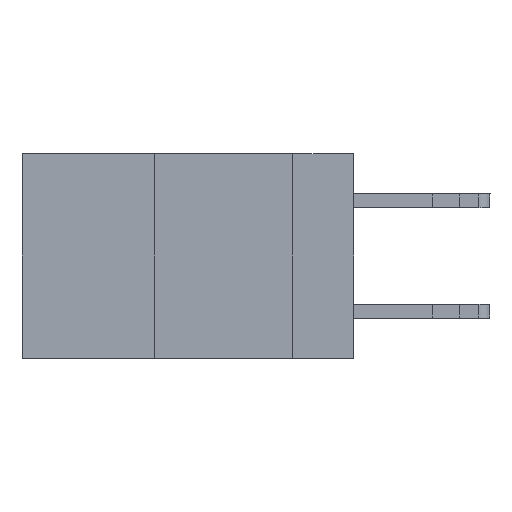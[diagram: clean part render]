
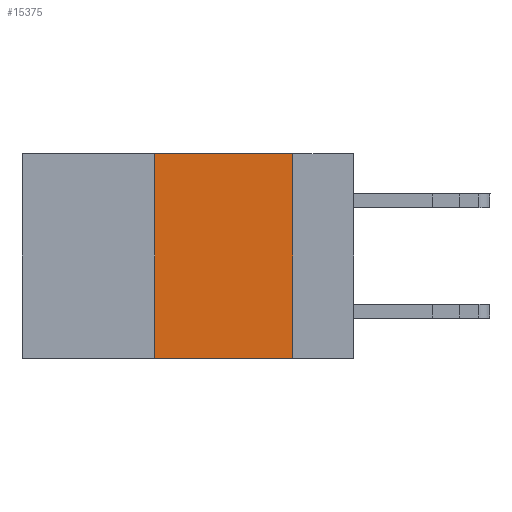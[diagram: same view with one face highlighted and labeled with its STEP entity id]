
A CAD part, left-side view. The second image highlights one B-rep face of the part: STEP entity #15375.
In plain terms, the highlighted planar face has unit normal (-1, 0, 0).
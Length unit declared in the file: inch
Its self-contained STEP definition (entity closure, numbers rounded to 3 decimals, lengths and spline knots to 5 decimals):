
#1478 = EDGE_CURVE ( 'NONE', #24300, #24697, #26715, .T. ) ;
#2427 = EDGE_CURVE ( 'NONE', #22450, #24697, #25152, .T. ) ;
#2754 = CARTESIAN_POINT ( 'NONE',  ( 0., 0.11, 0. ) ) ;
#3565 = PLANE ( 'NONE',  #10828 ) ;
#3780 = DIRECTION ( 'NONE',  ( 1., 0., 0. ) ) ;
#5865 = DIRECTION ( 'NONE',  ( 0., 0., 1. ) ) ;
#6190 = DIRECTION ( 'NONE',  ( 0., 0., -1. ) ) ;
#7989 = VECTOR ( 'NONE', #25671, 39.37008 ) ;
#8071 = ORIENTED_EDGE ( 'NONE', *, *, #12324, .F. ) ;
#8124 = ORIENTED_EDGE ( 'NONE', *, *, #1478, .T. ) ;
#8428 = ORIENTED_EDGE ( 'NONE', *, *, #28635, .F. ) ;
#8718 = VECTOR ( 'NONE', #17264, 39.37008 ) ;
#10828 = AXIS2_PLACEMENT_3D ( 'NONE', #18059, #3780, #6190 ) ;
#11264 = CARTESIAN_POINT ( 'NONE',  ( 0., 0.36, 0. ) ) ;
#11958 = CARTESIAN_POINT ( 'NONE',  ( 0., 0.11, -0.37 ) ) ;
#12175 = CARTESIAN_POINT ( 'NONE',  ( 0., 0.36, 0. ) ) ;
#12324 = EDGE_CURVE ( 'NONE', #24300, #23163, #24740, .T. ) ;
#14173 = EDGE_LOOP ( 'NONE', ( #14242, #8428, #8071, #8124 ) ) ;
#14242 = ORIENTED_EDGE ( 'NONE', *, *, #2427, .F. ) ;
#15375 = ADVANCED_FACE ( 'NONE', ( #24974 ), #3565, .F. ) ;
#16295 = CARTESIAN_POINT ( 'NONE',  ( 0., 0.6, -0.37 ) ) ;
#17264 = DIRECTION ( 'NONE',  ( 0., -1., 0. ) ) ;
#17408 = CARTESIAN_POINT ( 'NONE',  ( 0., 0.36, -0.37 ) ) ;
#18059 = CARTESIAN_POINT ( 'NONE',  ( 0., 0.6, 0. ) ) ;
#18063 = VECTOR ( 'NONE', #22078, 39.37008 ) ;
#18240 = CARTESIAN_POINT ( 'NONE',  ( 0., 0.11, 0. ) ) ;
#22078 = DIRECTION ( 'NONE',  ( 0., 0., -1. ) ) ;
#22450 = VERTEX_POINT ( 'NONE', #18240 ) ;
#23163 = VERTEX_POINT ( 'NONE', #11264 ) ;
#24300 = VERTEX_POINT ( 'NONE', #17408 ) ;
#24556 = CARTESIAN_POINT ( 'NONE',  ( 0., 0.6, 0. ) ) ;
#24697 = VERTEX_POINT ( 'NONE', #11958 ) ;
#24740 = LINE ( 'NONE', #12175, #28860 ) ;
#24974 = FACE_OUTER_BOUND ( 'NONE', #14173, .T. ) ;
#25152 = LINE ( 'NONE', #2754, #18063 ) ;
#25597 = LINE ( 'NONE', #24556, #8718 ) ;
#25671 = DIRECTION ( 'NONE',  ( 0., -1., 0. ) ) ;
#26715 = LINE ( 'NONE', #16295, #7989 ) ;
#28635 = EDGE_CURVE ( 'NONE', #23163, #22450, #25597, .T. ) ;
#28860 = VECTOR ( 'NONE', #5865, 39.37008 ) ;
